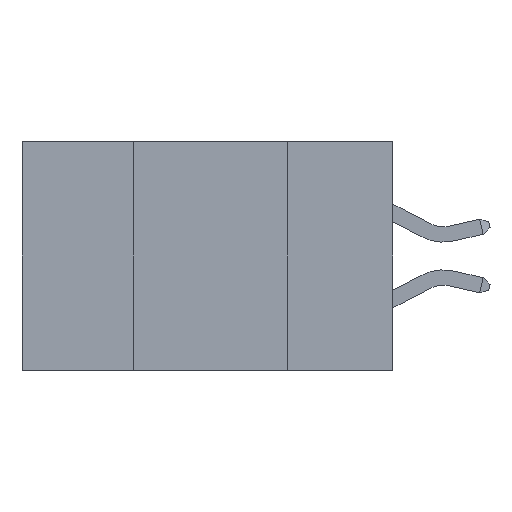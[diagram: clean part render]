
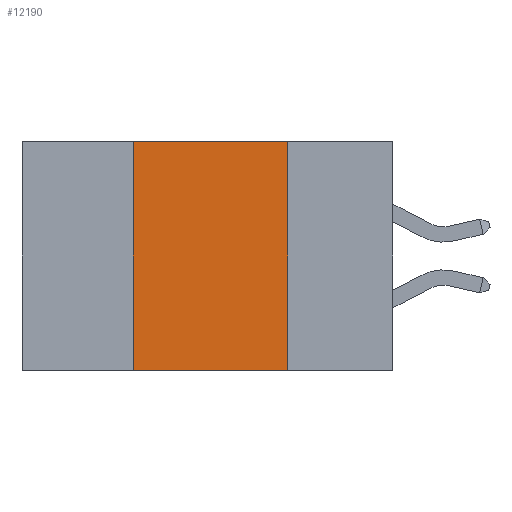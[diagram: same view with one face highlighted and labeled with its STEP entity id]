
A CAD part, left-side view. The second image highlights one B-rep face of the part: STEP entity #12190.
In plain terms, the highlighted planar face has unit normal (-1, 0, 0).
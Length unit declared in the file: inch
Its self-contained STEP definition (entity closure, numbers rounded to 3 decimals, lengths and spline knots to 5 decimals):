
#613 = ORIENTED_EDGE ( 'NONE', *, *, #1892, .F. ) ;
#1308 = VERTEX_POINT ( 'NONE', #19294 ) ;
#1892 = EDGE_CURVE ( 'NONE', #19848, #12470, #11760, .T. ) ;
#2490 = CARTESIAN_POINT ( 'NONE',  ( 0., 0.42, 0. ) ) ;
#3268 = AXIS2_PLACEMENT_3D ( 'NONE', #20056, #21744, #11455 ) ;
#3322 = VERTEX_POINT ( 'NONE', #12331 ) ;
#3608 = EDGE_CURVE ( 'NONE', #1308, #19848, #18970, .T. ) ;
#5477 = VECTOR ( 'NONE', #16682, 39.37008 ) ;
#6757 = FACE_OUTER_BOUND ( 'NONE', #7317, .T. ) ;
#7317 = EDGE_LOOP ( 'NONE', ( #613, #18380, #15542, #14758 ) ) ;
#8121 = PLANE ( 'NONE',  #3268 ) ;
#9372 = DIRECTION ( 'NONE',  ( 0., 0., 1. ) ) ;
#10918 = CARTESIAN_POINT ( 'NONE',  ( 0., 0.17, 0. ) ) ;
#11455 = DIRECTION ( 'NONE',  ( 0., 0., -1. ) ) ;
#11760 = LINE ( 'NONE', #17560, #13920 ) ;
#12190 = ADVANCED_FACE ( 'NONE', ( #6757 ), #8121, .F. ) ;
#12331 = CARTESIAN_POINT ( 'NONE',  ( 0., 0.42, -0.37 ) ) ;
#12470 = VERTEX_POINT ( 'NONE', #17780 ) ;
#12678 = DIRECTION ( 'NONE',  ( 0., -1., 0. ) ) ;
#12888 = DIRECTION ( 'NONE',  ( 0., 0., -1. ) ) ;
#13644 = CARTESIAN_POINT ( 'NONE',  ( 0., 0.6, 0. ) ) ;
#13920 = VECTOR ( 'NONE', #12888, 39.37008 ) ;
#14459 = VECTOR ( 'NONE', #9372, 39.37008 ) ;
#14758 = ORIENTED_EDGE ( 'NONE', *, *, #21849, .T. ) ;
#15462 = VECTOR ( 'NONE', #12678, 39.37008 ) ;
#15542 = ORIENTED_EDGE ( 'NONE', *, *, #18223, .F. ) ;
#16682 = DIRECTION ( 'NONE',  ( 0., -1., 0. ) ) ;
#16866 = LINE ( 'NONE', #2490, #14459 ) ;
#17560 = CARTESIAN_POINT ( 'NONE',  ( 0., 0.17, 0. ) ) ;
#17780 = CARTESIAN_POINT ( 'NONE',  ( 0., 0.17, -0.37 ) ) ;
#18223 = EDGE_CURVE ( 'NONE', #3322, #1308, #16866, .T. ) ;
#18380 = ORIENTED_EDGE ( 'NONE', *, *, #3608, .F. ) ;
#18709 = CARTESIAN_POINT ( 'NONE',  ( 0., 0.6, -0.37 ) ) ;
#18970 = LINE ( 'NONE', #13644, #15462 ) ;
#19134 = LINE ( 'NONE', #18709, #5477 ) ;
#19294 = CARTESIAN_POINT ( 'NONE',  ( 0., 0.42, 0. ) ) ;
#19848 = VERTEX_POINT ( 'NONE', #10918 ) ;
#20056 = CARTESIAN_POINT ( 'NONE',  ( 0., 0.6, 0. ) ) ;
#21744 = DIRECTION ( 'NONE',  ( 1., 0., 0. ) ) ;
#21849 = EDGE_CURVE ( 'NONE', #3322, #12470, #19134, .T. ) ;
